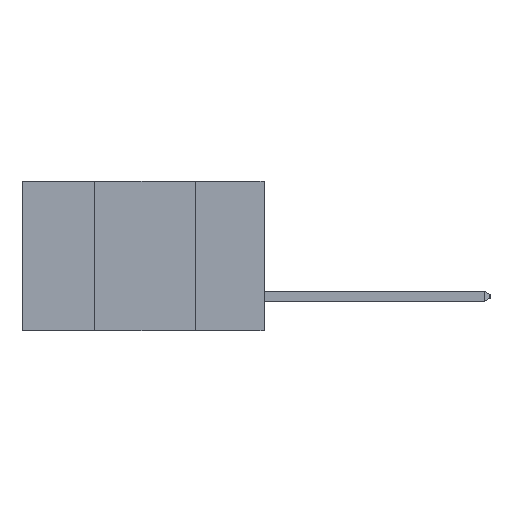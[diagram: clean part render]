
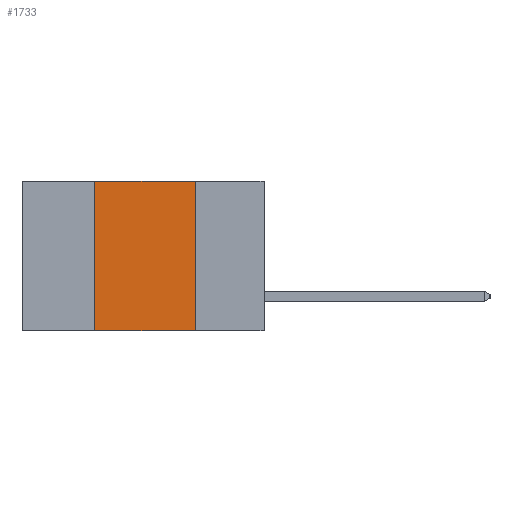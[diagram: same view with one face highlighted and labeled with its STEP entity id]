
A CAD part, left-side view. The second image highlights one B-rep face of the part: STEP entity #1733.
In plain terms, the highlighted planar face has unit normal (-1, 0, 0).
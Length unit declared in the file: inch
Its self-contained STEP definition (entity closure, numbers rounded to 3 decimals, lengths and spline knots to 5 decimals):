
#200 = VECTOR ( 'NONE', #7079, 39.37008 ) ;
#853 = CARTESIAN_POINT ( 'NONE',  ( 0., 0.17, -0.37 ) ) ;
#922 = VECTOR ( 'NONE', #13030, 39.37008 ) ;
#1091 = VECTOR ( 'NONE', #11333, 39.37008 ) ;
#1134 = EDGE_CURVE ( 'NONE', #8582, #2014, #5757, .T. ) ;
#1733 = ADVANCED_FACE ( 'NONE', ( #6894 ), #4957, .F. ) ;
#2014 = VERTEX_POINT ( 'NONE', #853 ) ;
#2375 = CARTESIAN_POINT ( 'NONE',  ( 0., 0.17, 0. ) ) ;
#2478 = ORIENTED_EDGE ( 'NONE', *, *, #10385, .F. ) ;
#2573 = VERTEX_POINT ( 'NONE', #4941 ) ;
#4037 = EDGE_LOOP ( 'NONE', ( #9077, #11078, #2478, #5327 ) ) ;
#4222 = CARTESIAN_POINT ( 'NONE',  ( 0., 0.6, 0. ) ) ;
#4723 = EDGE_CURVE ( 'NONE', #2573, #11274, #12090, .T. ) ;
#4872 = CARTESIAN_POINT ( 'NONE',  ( 0., 0.42, -0.37 ) ) ;
#4941 = CARTESIAN_POINT ( 'NONE',  ( 0., 0.42, 0. ) ) ;
#4957 = PLANE ( 'NONE',  #8851 ) ;
#5327 = ORIENTED_EDGE ( 'NONE', *, *, #1134, .T. ) ;
#5757 = LINE ( 'NONE', #6722, #200 ) ;
#5810 = CARTESIAN_POINT ( 'NONE',  ( 0., 0.42, -0.37 ) ) ;
#5873 = LINE ( 'NONE', #6843, #10767 ) ;
#6722 = CARTESIAN_POINT ( 'NONE',  ( 0., 0.6, -0.37 ) ) ;
#6827 = LINE ( 'NONE', #4872, #922 ) ;
#6843 = CARTESIAN_POINT ( 'NONE',  ( 0., 0.17, -0.37 ) ) ;
#6887 = DIRECTION ( 'NONE',  ( 0., 0., -1. ) ) ;
#6894 = FACE_OUTER_BOUND ( 'NONE', #4037, .T. ) ;
#7079 = DIRECTION ( 'NONE',  ( 0., -1., 0. ) ) ;
#8474 = EDGE_CURVE ( 'NONE', #11274, #2014, #5873, .T. ) ;
#8582 = VERTEX_POINT ( 'NONE', #5810 ) ;
#8851 = AXIS2_PLACEMENT_3D ( 'NONE', #4222, #9374, #10310 ) ;
#9077 = ORIENTED_EDGE ( 'NONE', *, *, #8474, .F. ) ;
#9374 = DIRECTION ( 'NONE',  ( 1., 0., 0. ) ) ;
#10310 = DIRECTION ( 'NONE',  ( 0., 0., -1. ) ) ;
#10385 = EDGE_CURVE ( 'NONE', #8582, #2573, #6827, .T. ) ;
#10767 = VECTOR ( 'NONE', #6887, 39.37008 ) ;
#11078 = ORIENTED_EDGE ( 'NONE', *, *, #4723, .F. ) ;
#11186 = CARTESIAN_POINT ( 'NONE',  ( 0., 0.6, 0. ) ) ;
#11274 = VERTEX_POINT ( 'NONE', #2375 ) ;
#11333 = DIRECTION ( 'NONE',  ( 0., -1., 0. ) ) ;
#12090 = LINE ( 'NONE', #11186, #1091 ) ;
#13030 = DIRECTION ( 'NONE',  ( 0., 0., 1. ) ) ;
